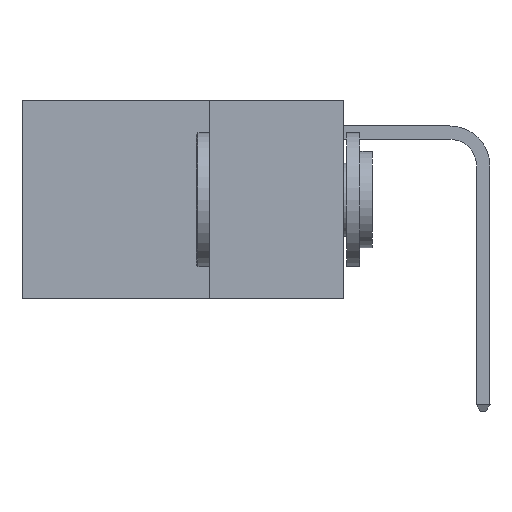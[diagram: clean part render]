
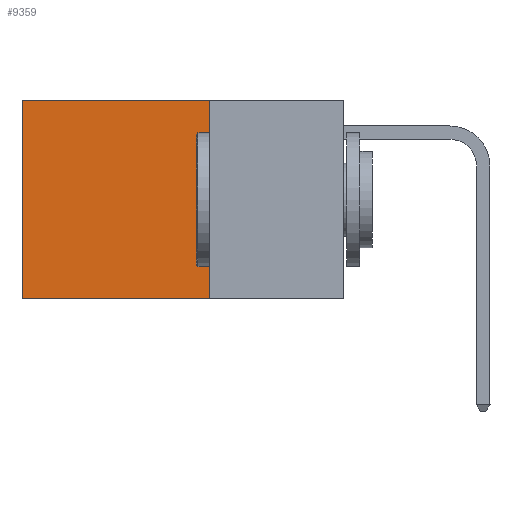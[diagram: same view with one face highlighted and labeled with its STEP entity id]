
A CAD part, left-side view. The second image highlights one B-rep face of the part: STEP entity #9359.
In plain terms, the highlighted planar face has unit normal (-1, 0, 0).
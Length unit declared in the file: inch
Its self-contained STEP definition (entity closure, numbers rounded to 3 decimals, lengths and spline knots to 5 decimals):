
#199 = CARTESIAN_POINT ( 'NONE',  ( 0.2625, 0.25, 0. ) ) ;
#262 = ORIENTED_EDGE ( 'NONE', *, *, #4962, .F. ) ;
#393 = VECTOR ( 'NONE', #1546, 39.37008 ) ;
#947 = CARTESIAN_POINT ( 'NONE',  ( 0.2625, 0.25, -0.37 ) ) ;
#1252 = DIRECTION ( 'NONE',  ( 0., 0., -1. ) ) ;
#1546 = DIRECTION ( 'NONE',  ( 0., 0., -1. ) ) ;
#1833 = FACE_OUTER_BOUND ( 'NONE', #9430, .T. ) ;
#2385 = DIRECTION ( 'NONE',  ( 0., 1., 0. ) ) ;
#2548 = EDGE_CURVE ( 'NONE', #9640, #6380, #4282, .T. ) ;
#2900 = VERTEX_POINT ( 'NONE', #947 ) ;
#2965 = LINE ( 'NONE', #4536, #393 ) ;
#3414 = EDGE_CURVE ( 'NONE', #2900, #6380, #9724, .T. ) ;
#3755 = ORIENTED_EDGE ( 'NONE', *, *, #3414, .F. ) ;
#3897 = AXIS2_PLACEMENT_3D ( 'NONE', #199, #7118, #3942 ) ;
#3942 = DIRECTION ( 'NONE',  ( 0., 0., -1. ) ) ;
#4282 = LINE ( 'NONE', #6525, #8483 ) ;
#4343 = VECTOR ( 'NONE', #2385, 39.37008 ) ;
#4536 = CARTESIAN_POINT ( 'NONE',  ( 0.2625, 0.25, 0. ) ) ;
#4784 = CARTESIAN_POINT ( 'NONE',  ( 0.2625, 0.25, 0. ) ) ;
#4962 = EDGE_CURVE ( 'NONE', #7272, #2900, #2965, .T. ) ;
#5092 = CARTESIAN_POINT ( 'NONE',  ( 0.2625, 0.25, -0.37 ) ) ;
#5548 = CARTESIAN_POINT ( 'NONE',  ( 0.2625, 0.25, 0. ) ) ;
#5865 = ORIENTED_EDGE ( 'NONE', *, *, #2548, .T. ) ;
#6380 = VERTEX_POINT ( 'NONE', #7746 ) ;
#6437 = EDGE_CURVE ( 'NONE', #7272, #9640, #7705, .T. ) ;
#6499 = VECTOR ( 'NONE', #6690, 39.37008 ) ;
#6525 = CARTESIAN_POINT ( 'NONE',  ( 0.2625, 0.6, 0. ) ) ;
#6690 = DIRECTION ( 'NONE',  ( 0., 1., 0. ) ) ;
#6780 = CARTESIAN_POINT ( 'NONE',  ( 0.2625, 0.6, 0. ) ) ;
#7118 = DIRECTION ( 'NONE',  ( 1., 0., 0. ) ) ;
#7272 = VERTEX_POINT ( 'NONE', #5548 ) ;
#7705 = LINE ( 'NONE', #4784, #4343 ) ;
#7746 = CARTESIAN_POINT ( 'NONE',  ( 0.2625, 0.6, -0.37 ) ) ;
#7844 = PLANE ( 'NONE',  #3897 ) ;
#8483 = VECTOR ( 'NONE', #1252, 39.37008 ) ;
#9169 = ORIENTED_EDGE ( 'NONE', *, *, #6437, .T. ) ;
#9359 = ADVANCED_FACE ( 'NONE', ( #1833 ), #7844, .F. ) ;
#9430 = EDGE_LOOP ( 'NONE', ( #5865, #3755, #262, #9169 ) ) ;
#9640 = VERTEX_POINT ( 'NONE', #6780 ) ;
#9724 = LINE ( 'NONE', #5092, #6499 ) ;
